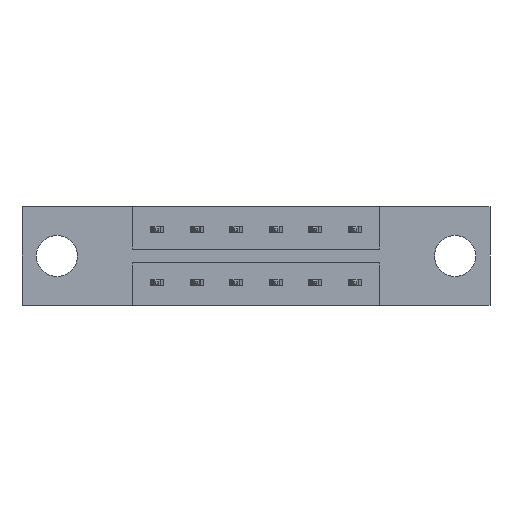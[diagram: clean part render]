
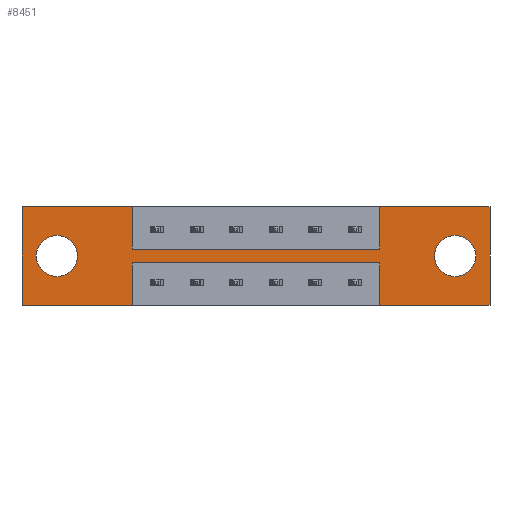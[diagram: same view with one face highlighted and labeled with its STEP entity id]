
A CAD part, front view. The second image highlights one B-rep face of the part: STEP entity #8451.
In plain terms, the highlighted planar face has unit normal (0, -1, 0).
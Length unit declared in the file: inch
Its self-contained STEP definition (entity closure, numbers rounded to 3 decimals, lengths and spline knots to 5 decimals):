
#64 = DIRECTION ( 'NONE',  ( 1., 0., 0. ) ) ;
#72 = LINE ( 'NONE', #4636, #5031 ) ;
#119 = VERTEX_POINT ( 'NONE', #5173 ) ;
#147 = VECTOR ( 'NONE', #7222, 39.37008 ) ;
#155 = DIRECTION ( 'NONE',  ( 0., 0., 1. ) ) ;
#176 = EDGE_CURVE ( 'NONE', #3941, #558, #4841, .T. ) ;
#306 = CARTESIAN_POINT ( 'NONE',  ( 1.6425, 0., -0.2655 ) ) ;
#325 = FACE_BOUND ( 'NONE', #6835, .T. ) ;
#399 = DIRECTION ( 'NONE',  ( -1., 0., 0. ) ) ;
#452 = VECTOR ( 'NONE', #5984, 39.37008 ) ;
#474 = EDGE_CURVE ( 'NONE', #5844, #1400, #8329, .T. ) ;
#528 = CARTESIAN_POINT ( 'NONE',  ( 1.775, 0., -0.375 ) ) ;
#558 = VERTEX_POINT ( 'NONE', #6559 ) ;
#656 = LINE ( 'NONE', #7619, #4896 ) ;
#664 = EDGE_CURVE ( 'NONE', #4180, #7522, #8095, .T. ) ;
#704 = VECTOR ( 'NONE', #8386, 39.37008 ) ;
#715 = VERTEX_POINT ( 'NONE', #6103 ) ;
#968 = DIRECTION ( 'NONE',  ( 0., 0., -1. ) ) ;
#1012 = EDGE_CURVE ( 'NONE', #558, #715, #8275, .T. ) ;
#1078 = CARTESIAN_POINT ( 'NONE',  ( 1.6425, 0., -0.1875 ) ) ;
#1088 = CARTESIAN_POINT ( 'NONE',  ( 0.1325, 0., -0.1095 ) ) ;
#1203 = DIRECTION ( 'NONE',  ( 0., 1., 0. ) ) ;
#1235 = LINE ( 'NONE', #4528, #704 ) ;
#1247 = VERTEX_POINT ( 'NONE', #3211 ) ;
#1261 = DIRECTION ( 'NONE',  ( 0., 0., 1. ) ) ;
#1264 = CARTESIAN_POINT ( 'NONE',  ( 0.1325, 0., -0.1875 ) ) ;
#1351 = EDGE_CURVE ( 'NONE', #1400, #5844, #5154, .T. ) ;
#1400 = VERTEX_POINT ( 'NONE', #8112 ) ;
#1479 = CARTESIAN_POINT ( 'NONE',  ( 0., 0., 0. ) ) ;
#1529 = CARTESIAN_POINT ( 'NONE',  ( 0.4175, 0., -0.375 ) ) ;
#1560 = ORIENTED_EDGE ( 'NONE', *, *, #3145, .T. ) ;
#1579 = ORIENTED_EDGE ( 'NONE', *, *, #474, .T. ) ;
#1653 = VERTEX_POINT ( 'NONE', #5863 ) ;
#1938 = LINE ( 'NONE', #4558, #6059 ) ;
#2014 = ORIENTED_EDGE ( 'NONE', *, *, #7852, .F. ) ;
#2047 = LINE ( 'NONE', #5785, #147 ) ;
#2125 = CARTESIAN_POINT ( 'NONE',  ( 1.6425, 0., -0.1095 ) ) ;
#2332 = ORIENTED_EDGE ( 'NONE', *, *, #4580, .F. ) ;
#2406 = AXIS2_PLACEMENT_3D ( 'NONE', #1264, #1203, #8448 ) ;
#2474 = ORIENTED_EDGE ( 'NONE', *, *, #3967, .F. ) ;
#2491 = DIRECTION ( 'NONE',  ( 0., 1., 0. ) ) ;
#2560 = ORIENTED_EDGE ( 'NONE', *, *, #3566, .F. ) ;
#2677 = EDGE_CURVE ( 'NONE', #7877, #4237, #5967, .T. ) ;
#2894 = EDGE_CURVE ( 'NONE', #7979, #5587, #6470, .T. ) ;
#3145 = EDGE_CURVE ( 'NONE', #4237, #7877, #6580, .T. ) ;
#3170 = VECTOR ( 'NONE', #5804, 39.37008 ) ;
#3211 = CARTESIAN_POINT ( 'NONE',  ( 0.4175, 0., 0. ) ) ;
#3414 = VECTOR ( 'NONE', #399, 39.37008 ) ;
#3491 = EDGE_LOOP ( 'NONE', ( #1579, #6691 ) ) ;
#3541 = CARTESIAN_POINT ( 'NONE',  ( 0., 0., -0.375 ) ) ;
#3566 = EDGE_CURVE ( 'NONE', #1653, #119, #3751, .T. ) ;
#3569 = LINE ( 'NONE', #3800, #3170 ) ;
#3751 = LINE ( 'NONE', #6182, #6668 ) ;
#3799 = CARTESIAN_POINT ( 'NONE',  ( 1.3575, 0., -0.214 ) ) ;
#3800 = CARTESIAN_POINT ( 'NONE',  ( 0.4175, 0., -0.161 ) ) ;
#3859 = DIRECTION ( 'NONE',  ( 0., 1., 0. ) ) ;
#3941 = VERTEX_POINT ( 'NONE', #4059 ) ;
#3967 = EDGE_CURVE ( 'NONE', #5587, #1247, #7562, .T. ) ;
#3990 = CARTESIAN_POINT ( 'NONE',  ( 0.1325, 0., -0.1875 ) ) ;
#4048 = CARTESIAN_POINT ( 'NONE',  ( 0., 0., 0. ) ) ;
#4059 = CARTESIAN_POINT ( 'NONE',  ( 1.3575, 0., -0.375 ) ) ;
#4139 = ORIENTED_EDGE ( 'NONE', *, *, #1012, .F. ) ;
#4180 = VERTEX_POINT ( 'NONE', #7105 ) ;
#4237 = VERTEX_POINT ( 'NONE', #2125 ) ;
#4354 = DIRECTION ( 'NONE',  ( 1., 0., 0. ) ) ;
#4397 = VECTOR ( 'NONE', #6504, 39.37008 ) ;
#4528 = CARTESIAN_POINT ( 'NONE',  ( 0., 0., -0.375 ) ) ;
#4548 = CARTESIAN_POINT ( 'NONE',  ( 0., 0., 0. ) ) ;
#4558 = CARTESIAN_POINT ( 'NONE',  ( 0., 0., -0.375 ) ) ;
#4580 = EDGE_CURVE ( 'NONE', #7522, #7517, #2047, .T. ) ;
#4636 = CARTESIAN_POINT ( 'NONE',  ( 0.4175, 0., -0.214 ) ) ;
#4841 = LINE ( 'NONE', #3799, #4397 ) ;
#4868 = DIRECTION ( 'NONE',  ( 0., -1., 0. ) ) ;
#4896 = VECTOR ( 'NONE', #7591, 39.37008 ) ;
#4925 = VECTOR ( 'NONE', #1261, 39.37008 ) ;
#5031 = VECTOR ( 'NONE', #6639, 39.37008 ) ;
#5154 = CIRCLE ( 'NONE', #6220, 0.078 ) ;
#5157 = CARTESIAN_POINT ( 'NONE',  ( 0.4175, 0., -0.214 ) ) ;
#5173 = CARTESIAN_POINT ( 'NONE',  ( 1.3575, 0., -0.161 ) ) ;
#5221 = EDGE_CURVE ( 'NONE', #1247, #1653, #3569, .T. ) ;
#5262 = EDGE_CURVE ( 'NONE', #7237, #7979, #1235, .T. ) ;
#5371 = ORIENTED_EDGE ( 'NONE', *, *, #5221, .F. ) ;
#5413 = FACE_OUTER_BOUND ( 'NONE', #6375, .T. ) ;
#5415 = ORIENTED_EDGE ( 'NONE', *, *, #2894, .F. ) ;
#5587 = VERTEX_POINT ( 'NONE', #8137 ) ;
#5589 = PLANE ( 'NONE',  #6293 ) ;
#5679 = AXIS2_PLACEMENT_3D ( 'NONE', #1078, #2491, #7103 ) ;
#5785 = CARTESIAN_POINT ( 'NONE',  ( 1.775, 0., 0. ) ) ;
#5804 = DIRECTION ( 'NONE',  ( 0., 0., -1. ) ) ;
#5844 = VERTEX_POINT ( 'NONE', #1088 ) ;
#5863 = CARTESIAN_POINT ( 'NONE',  ( 0.4175, 0., -0.161 ) ) ;
#5926 = DIRECTION ( 'NONE',  ( -1., 0., 0. ) ) ;
#5929 = DIRECTION ( 'NONE',  ( 0., 0., -1. ) ) ;
#5967 = CIRCLE ( 'NONE', #7756, 0.078 ) ;
#5984 = DIRECTION ( 'NONE',  ( 1., 0., 0. ) ) ;
#6059 = VECTOR ( 'NONE', #5926, 39.37008 ) ;
#6103 = CARTESIAN_POINT ( 'NONE',  ( 0.4175, 0., -0.214 ) ) ;
#6182 = CARTESIAN_POINT ( 'NONE',  ( 0.4175, 0., -0.161 ) ) ;
#6220 = AXIS2_PLACEMENT_3D ( 'NONE', #3990, #7993, #155 ) ;
#6222 = EDGE_CURVE ( 'NONE', #715, #7237, #72, .T. ) ;
#6293 = AXIS2_PLACEMENT_3D ( 'NONE', #3541, #4868, #968 ) ;
#6339 = ORIENTED_EDGE ( 'NONE', *, *, #2677, .T. ) ;
#6363 = ORIENTED_EDGE ( 'NONE', *, *, #5262, .F. ) ;
#6375 = EDGE_LOOP ( 'NONE', ( #7672, #7918, #2332, #7573, #2014, #2560, #5371, #2474, #5415, #6363, #6743, #4139 ) ) ;
#6428 = CARTESIAN_POINT ( 'NONE',  ( 0., 0., -0.375 ) ) ;
#6470 = LINE ( 'NONE', #4548, #4925 ) ;
#6504 = DIRECTION ( 'NONE',  ( 0., 0., 1. ) ) ;
#6559 = CARTESIAN_POINT ( 'NONE',  ( 1.3575, 0., -0.214 ) ) ;
#6580 = CIRCLE ( 'NONE', #5679, 0.078 ) ;
#6639 = DIRECTION ( 'NONE',  ( 0., 0., -1. ) ) ;
#6649 = FACE_BOUND ( 'NONE', #3491, .T. ) ;
#6668 = VECTOR ( 'NONE', #4354, 39.37008 ) ;
#6691 = ORIENTED_EDGE ( 'NONE', *, *, #1351, .T. ) ;
#6743 = ORIENTED_EDGE ( 'NONE', *, *, #6222, .F. ) ;
#6810 = EDGE_CURVE ( 'NONE', #7517, #3941, #1938, .T. ) ;
#6835 = EDGE_LOOP ( 'NONE', ( #1560, #6339 ) ) ;
#7006 = CARTESIAN_POINT ( 'NONE',  ( 1.775, 0., 0. ) ) ;
#7103 = DIRECTION ( 'NONE',  ( 0., 0., -1. ) ) ;
#7105 = CARTESIAN_POINT ( 'NONE',  ( 1.3575, 0., 0. ) ) ;
#7189 = CARTESIAN_POINT ( 'NONE',  ( 1.6425, 0., -0.1875 ) ) ;
#7222 = DIRECTION ( 'NONE',  ( 0., 0., -1. ) ) ;
#7237 = VERTEX_POINT ( 'NONE', #1529 ) ;
#7377 = VECTOR ( 'NONE', #64, 39.37008 ) ;
#7517 = VERTEX_POINT ( 'NONE', #528 ) ;
#7522 = VERTEX_POINT ( 'NONE', #7006 ) ;
#7562 = LINE ( 'NONE', #1479, #7377 ) ;
#7573 = ORIENTED_EDGE ( 'NONE', *, *, #664, .F. ) ;
#7591 = DIRECTION ( 'NONE',  ( 0., 0., 1. ) ) ;
#7619 = CARTESIAN_POINT ( 'NONE',  ( 1.3575, 0., -0.161 ) ) ;
#7672 = ORIENTED_EDGE ( 'NONE', *, *, #176, .F. ) ;
#7756 = AXIS2_PLACEMENT_3D ( 'NONE', #7189, #3859, #5929 ) ;
#7852 = EDGE_CURVE ( 'NONE', #119, #4180, #656, .T. ) ;
#7877 = VERTEX_POINT ( 'NONE', #306 ) ;
#7918 = ORIENTED_EDGE ( 'NONE', *, *, #6810, .F. ) ;
#7979 = VERTEX_POINT ( 'NONE', #6428 ) ;
#7993 = DIRECTION ( 'NONE',  ( 0., 1., 0. ) ) ;
#8095 = LINE ( 'NONE', #4048, #452 ) ;
#8112 = CARTESIAN_POINT ( 'NONE',  ( 0.1325, 0., -0.2655 ) ) ;
#8137 = CARTESIAN_POINT ( 'NONE',  ( 0., 0., 0. ) ) ;
#8275 = LINE ( 'NONE', #5157, #3414 ) ;
#8329 = CIRCLE ( 'NONE', #2406, 0.078 ) ;
#8386 = DIRECTION ( 'NONE',  ( -1., 0., 0. ) ) ;
#8448 = DIRECTION ( 'NONE',  ( 0., 0., 1. ) ) ;
#8451 = ADVANCED_FACE ( 'NONE', ( #325, #6649, #5413 ), #5589, .T. ) ;
